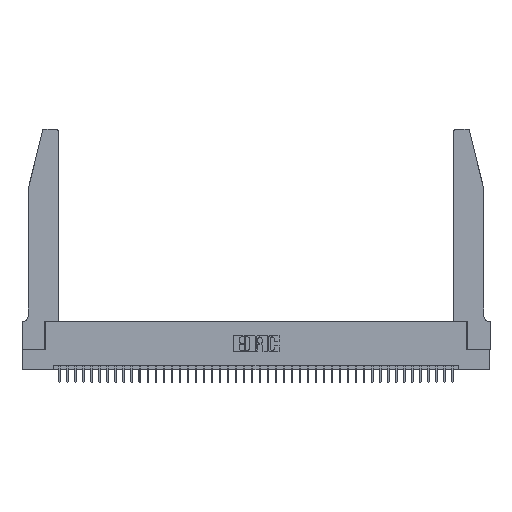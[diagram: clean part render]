
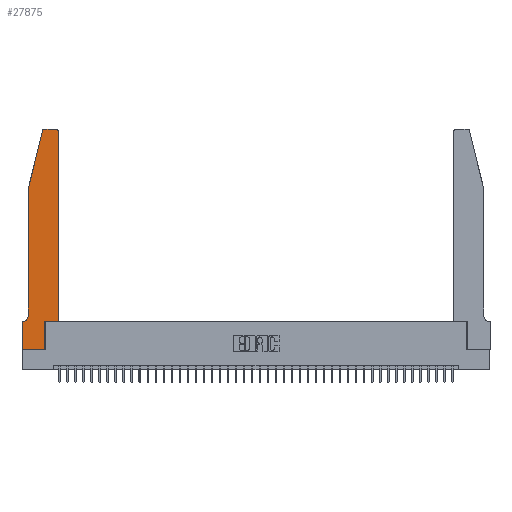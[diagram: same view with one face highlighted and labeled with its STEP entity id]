
A CAD part, top view. The second image highlights one B-rep face of the part: STEP entity #27875.
In plain terms, the highlighted planar face has unit normal (0, 0, 1).
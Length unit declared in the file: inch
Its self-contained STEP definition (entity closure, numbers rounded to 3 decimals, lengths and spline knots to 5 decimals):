
#216 = DIRECTION ( 'NONE',  ( 1., 0., 0. ) ) ;
#821 = VECTOR ( 'NONE', #16256, 39.37008 ) ;
#873 = CARTESIAN_POINT ( 'NONE',  ( 0.4505, 0.35, 0.37 ) ) ;
#1876 = LINE ( 'NONE', #39267, #821 ) ;
#2079 = CARTESIAN_POINT ( 'NONE',  ( 0.284, 2.75, 0.37 ) ) ;
#3335 = CARTESIAN_POINT ( 'NONE',  ( 0., 0.35, 0.37 ) ) ;
#4559 = EDGE_CURVE ( 'NONE', #18382, #33948, #20104, .T. ) ;
#4711 = EDGE_CURVE ( 'NONE', #37914, #10111, #14917, .T. ) ;
#5330 = VECTOR ( 'NONE', #24312, 39.37008 ) ;
#5341 = ORIENTED_EDGE ( 'NONE', *, *, #10768, .T. ) ;
#5424 = ORIENTED_EDGE ( 'NONE', *, *, #35850, .T. ) ;
#5527 = DIRECTION ( 'NONE',  ( 0., 0., -1. ) ) ;
#5922 = CARTESIAN_POINT ( 'NONE',  ( 0., 0., 0.37 ) ) ;
#6870 = CARTESIAN_POINT ( 'NONE',  ( 0., 0., 0.37 ) ) ;
#6961 = EDGE_CURVE ( 'NONE', #40689, #13428, #34642, .T. ) ;
#7032 = CARTESIAN_POINT ( 'NONE',  ( 0.4205, 2.75, 0.37 ) ) ;
#7373 = AXIS2_PLACEMENT_3D ( 'NONE', #40020, #20343, #216 ) ;
#7541 = DIRECTION ( 'NONE',  ( 0., 1., 0. ) ) ;
#8817 = CARTESIAN_POINT ( 'NONE',  ( 0., 0.35, 0.37 ) ) ;
#8952 = CARTESIAN_POINT ( 'NONE',  ( 0.2605, 2.75, 0.37 ) ) ;
#9288 = LINE ( 'NONE', #6870, #16075 ) ;
#9387 = ORIENTED_EDGE ( 'NONE', *, *, #30143, .T. ) ;
#9999 = ORIENTED_EDGE ( 'NONE', *, *, #33594, .T. ) ;
#10111 = VERTEX_POINT ( 'NONE', #19288 ) ;
#10768 = EDGE_CURVE ( 'NONE', #34567, #23694, #23632, .T. ) ;
#10995 = ORIENTED_EDGE ( 'NONE', *, *, #27259, .T. ) ;
#11132 = AXIS2_PLACEMENT_3D ( 'NONE', #19053, #42085, #22409 ) ;
#11440 = CARTESIAN_POINT ( 'NONE',  ( 0., 0., 0.37 ) ) ;
#12252 = CARTESIAN_POINT ( 'NONE',  ( 0.2865, 0., 0.37 ) ) ;
#13352 = DIRECTION ( 'NONE',  ( 0., -1., 0. ) ) ;
#13428 = VERTEX_POINT ( 'NONE', #26289 ) ;
#13431 = CARTESIAN_POINT ( 'NONE',  ( 0.0755, 2., 0.37 ) ) ;
#14136 = VERTEX_POINT ( 'NONE', #3335 ) ;
#14398 = CIRCLE ( 'NONE', #21358, 0.07 ) ;
#14917 = LINE ( 'NONE', #37881, #41184 ) ;
#15533 = DIRECTION ( 'NONE',  ( 1., 0., 0. ) ) ;
#15823 = ORIENTED_EDGE ( 'NONE', *, *, #6961, .T. ) ;
#16075 = VECTOR ( 'NONE', #13352, 39.37008 ) ;
#16256 = DIRECTION ( 'NONE',  ( -1., 0., 0. ) ) ;
#17781 = EDGE_CURVE ( 'NONE', #29011, #14136, #1876, .T. ) ;
#18078 = CIRCLE ( 'NONE', #7373, 0.03 ) ;
#18183 = DIRECTION ( 'NONE',  ( 0., -1., 0. ) ) ;
#18382 = VERTEX_POINT ( 'NONE', #27508 ) ;
#18959 = DIRECTION ( 'NONE',  ( 0., 1., 0. ) ) ;
#18987 = DIRECTION ( 'NONE',  ( -1., 0., 0. ) ) ;
#19053 = CARTESIAN_POINT ( 'NONE',  ( 0.284, 2.72, 0.37 ) ) ;
#19288 = CARTESIAN_POINT ( 'NONE',  ( 0.0755, 0.42, 0.37 ) ) ;
#19538 = EDGE_CURVE ( 'NONE', #33948, #36760, #18078, .T. ) ;
#20104 = LINE ( 'NONE', #33999, #36530 ) ;
#20236 = VERTEX_POINT ( 'NONE', #11440 ) ;
#20343 = DIRECTION ( 'NONE',  ( 0., 0., 1. ) ) ;
#20374 = EDGE_CURVE ( 'NONE', #10111, #29011, #14398, .T. ) ;
#20507 = CARTESIAN_POINT ( 'NONE',  ( 0.0755, 2., 0.37 ) ) ;
#20643 = ORIENTED_EDGE ( 'NONE', *, *, #4711, .T. ) ;
#21358 = AXIS2_PLACEMENT_3D ( 'NONE', #25470, #5527, #28805 ) ;
#21714 = EDGE_CURVE ( 'NONE', #23694, #18382, #39506, .T. ) ;
#22056 = PLANE ( 'NONE',  #32800 ) ;
#22409 = DIRECTION ( 'NONE',  ( 1., 0., 0. ) ) ;
#23632 = LINE ( 'NONE', #25607, #32349 ) ;
#23686 = VECTOR ( 'NONE', #18987, 39.37008 ) ;
#23694 = VERTEX_POINT ( 'NONE', #34034 ) ;
#24312 = DIRECTION ( 'NONE',  ( 1., 0., 0. ) ) ;
#25470 = CARTESIAN_POINT ( 'NONE',  ( 0.0055, 0.42, 0.37 ) ) ;
#25607 = CARTESIAN_POINT ( 'NONE',  ( 0.2865, 0.35, 0.37 ) ) ;
#25848 = DIRECTION ( 'NONE',  ( 1., 0., 0. ) ) ;
#26289 = CARTESIAN_POINT ( 'NONE',  ( 0.25487, 2.72718, 0.37 ) ) ;
#27151 = DIRECTION ( 'NONE',  ( -0.239, -0.971, 0. ) ) ;
#27259 = EDGE_CURVE ( 'NONE', #13428, #37914, #33684, .T. ) ;
#27508 = CARTESIAN_POINT ( 'NONE',  ( 0.4505, 0.35, 0.37 ) ) ;
#27875 = ADVANCED_FACE ( 'NONE', ( #35149 ), #22056, .T. ) ;
#28400 = ORIENTED_EDGE ( 'NONE', *, *, #4559, .T. ) ;
#28805 = DIRECTION ( 'NONE',  ( -1., 0., 0. ) ) ;
#29011 = VERTEX_POINT ( 'NONE', #41206 ) ;
#29719 = ORIENTED_EDGE ( 'NONE', *, *, #17781, .T. ) ;
#30143 = EDGE_CURVE ( 'NONE', #36760, #40689, #42179, .T. ) ;
#32349 = VECTOR ( 'NONE', #18959, 39.37008 ) ;
#32800 = AXIS2_PLACEMENT_3D ( 'NONE', #8817, #35217, #15533 ) ;
#32949 = VECTOR ( 'NONE', #25848, 39.37008 ) ;
#33002 = EDGE_LOOP ( 'NONE', ( #9387, #15823, #10995, #20643, #42387, #29719, #9999, #5424, #5341, #40682, #28400, #41433 ) ) ;
#33594 = EDGE_CURVE ( 'NONE', #14136, #20236, #9288, .T. ) ;
#33684 = LINE ( 'NONE', #20507, #40379 ) ;
#33948 = VERTEX_POINT ( 'NONE', #34875 ) ;
#33999 = CARTESIAN_POINT ( 'NONE',  ( 0.4505, 0.35, 0.37 ) ) ;
#34034 = CARTESIAN_POINT ( 'NONE',  ( 0.2865, 0.35, 0.37 ) ) ;
#34567 = VERTEX_POINT ( 'NONE', #12252 ) ;
#34642 = CIRCLE ( 'NONE', #11132, 0.03 ) ;
#34875 = CARTESIAN_POINT ( 'NONE',  ( 0.4505, 2.72, 0.37 ) ) ;
#35149 = FACE_OUTER_BOUND ( 'NONE', #33002, .T. ) ;
#35217 = DIRECTION ( 'NONE',  ( 0., 0., 1. ) ) ;
#35850 = EDGE_CURVE ( 'NONE', #20236, #34567, #41701, .T. ) ;
#36530 = VECTOR ( 'NONE', #7541, 39.37008 ) ;
#36760 = VERTEX_POINT ( 'NONE', #7032 ) ;
#37881 = CARTESIAN_POINT ( 'NONE',  ( 0.0755, 2., 0.37 ) ) ;
#37914 = VERTEX_POINT ( 'NONE', #13431 ) ;
#39267 = CARTESIAN_POINT ( 'NONE',  ( 0.0755, 0.35, 0.37 ) ) ;
#39506 = LINE ( 'NONE', #873, #5330 ) ;
#40020 = CARTESIAN_POINT ( 'NONE',  ( 0.4205, 2.72, 0.37 ) ) ;
#40379 = VECTOR ( 'NONE', #27151, 39.37008 ) ;
#40682 = ORIENTED_EDGE ( 'NONE', *, *, #21714, .T. ) ;
#40689 = VERTEX_POINT ( 'NONE', #2079 ) ;
#41184 = VECTOR ( 'NONE', #18183, 39.37008 ) ;
#41206 = CARTESIAN_POINT ( 'NONE',  ( 0.0055, 0.35, 0.37 ) ) ;
#41433 = ORIENTED_EDGE ( 'NONE', *, *, #19538, .T. ) ;
#41701 = LINE ( 'NONE', #5922, #32949 ) ;
#42085 = DIRECTION ( 'NONE',  ( 0., 0., 1. ) ) ;
#42179 = LINE ( 'NONE', #8952, #23686 ) ;
#42387 = ORIENTED_EDGE ( 'NONE', *, *, #20374, .T. ) ;
